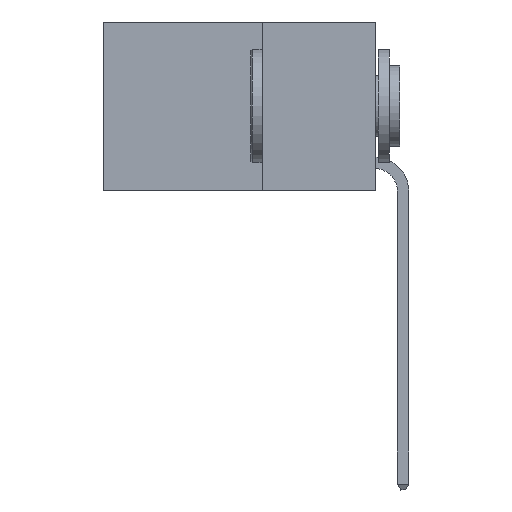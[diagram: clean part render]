
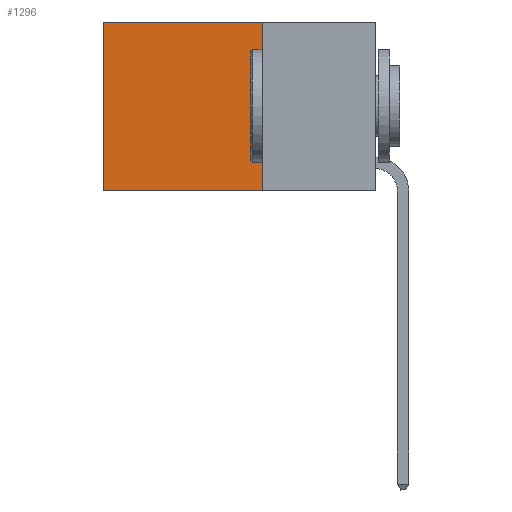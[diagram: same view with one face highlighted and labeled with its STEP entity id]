
A CAD part, left-side view. The second image highlights one B-rep face of the part: STEP entity #1296.
In plain terms, the highlighted planar face has unit normal (-1, 0, 0).
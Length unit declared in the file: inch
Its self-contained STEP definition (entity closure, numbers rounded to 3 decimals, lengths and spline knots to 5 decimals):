
#1296 = ADVANCED_FACE ( 'NONE', ( #5413 ), #10723, .F. ) ;
#1935 = EDGE_CURVE ( 'NONE', #15682, #12497, #5593, .T. ) ;
#3690 = CARTESIAN_POINT ( 'NONE',  ( 0.2625, 0.25, 0. ) ) ;
#4337 = LINE ( 'NONE', #12897, #13714 ) ;
#4672 = CARTESIAN_POINT ( 'NONE',  ( 0.2625, 0.6, 0. ) ) ;
#4890 = VECTOR ( 'NONE', #5494, 39.37008 ) ;
#5413 = FACE_OUTER_BOUND ( 'NONE', #21743, .T. ) ;
#5494 = DIRECTION ( 'NONE',  ( 0., 1., 0. ) ) ;
#5593 = LINE ( 'NONE', #5709, #4890 ) ;
#5709 = CARTESIAN_POINT ( 'NONE',  ( 0.2625, 0.25, 0. ) ) ;
#6687 = EDGE_CURVE ( 'NONE', #15682, #9173, #11525, .T. ) ;
#9007 = DIRECTION ( 'NONE',  ( 0., 0., -1. ) ) ;
#9173 = VERTEX_POINT ( 'NONE', #14268 ) ;
#9266 = ORIENTED_EDGE ( 'NONE', *, *, #1935, .T. ) ;
#9319 = ORIENTED_EDGE ( 'NONE', *, *, #16613, .T. ) ;
#9562 = EDGE_CURVE ( 'NONE', #9173, #14211, #4337, .T. ) ;
#9605 = VECTOR ( 'NONE', #13701, 39.37008 ) ;
#9690 = CARTESIAN_POINT ( 'NONE',  ( 0.2625, 0.25, 0. ) ) ;
#10723 = PLANE ( 'NONE',  #18227 ) ;
#11525 = LINE ( 'NONE', #9690, #20479 ) ;
#12497 = VERTEX_POINT ( 'NONE', #13634 ) ;
#12897 = CARTESIAN_POINT ( 'NONE',  ( 0.2625, 0.25, -0.37 ) ) ;
#13634 = CARTESIAN_POINT ( 'NONE',  ( 0.2625, 0.6, 0. ) ) ;
#13701 = DIRECTION ( 'NONE',  ( 0., 0., -1. ) ) ;
#13714 = VECTOR ( 'NONE', #19951, 39.37008 ) ;
#14211 = VERTEX_POINT ( 'NONE', #22453 ) ;
#14268 = CARTESIAN_POINT ( 'NONE',  ( 0.2625, 0.25, -0.37 ) ) ;
#15682 = VERTEX_POINT ( 'NONE', #18868 ) ;
#16073 = ORIENTED_EDGE ( 'NONE', *, *, #9562, .F. ) ;
#16613 = EDGE_CURVE ( 'NONE', #12497, #14211, #18800, .T. ) ;
#17786 = DIRECTION ( 'NONE',  ( 1., 0., 0. ) ) ;
#18227 = AXIS2_PLACEMENT_3D ( 'NONE', #3690, #17786, #9007 ) ;
#18800 = LINE ( 'NONE', #4672, #9605 ) ;
#18868 = CARTESIAN_POINT ( 'NONE',  ( 0.2625, 0.25, 0. ) ) ;
#19951 = DIRECTION ( 'NONE',  ( 0., 1., 0. ) ) ;
#20330 = ORIENTED_EDGE ( 'NONE', *, *, #6687, .F. ) ;
#20476 = DIRECTION ( 'NONE',  ( 0., 0., -1. ) ) ;
#20479 = VECTOR ( 'NONE', #20476, 39.37008 ) ;
#21743 = EDGE_LOOP ( 'NONE', ( #9319, #16073, #20330, #9266 ) ) ;
#22453 = CARTESIAN_POINT ( 'NONE',  ( 0.2625, 0.6, -0.37 ) ) ;
